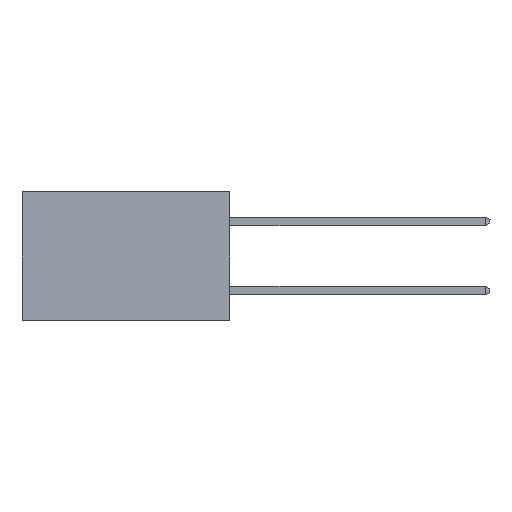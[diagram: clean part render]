
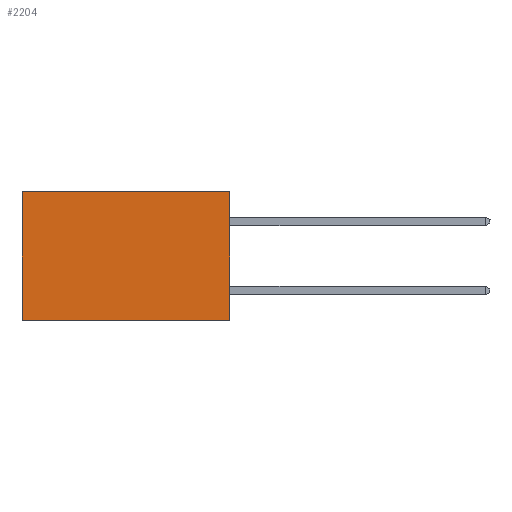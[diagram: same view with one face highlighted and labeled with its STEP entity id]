
A CAD part, left-side view. The second image highlights one B-rep face of the part: STEP entity #2204.
In plain terms, the highlighted planar face has unit normal (-1, 0, 0).
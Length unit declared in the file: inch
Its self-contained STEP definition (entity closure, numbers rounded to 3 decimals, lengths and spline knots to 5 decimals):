
#686 = CARTESIAN_POINT ( 'NONE',  ( 0.2615, 0., -0.37 ) ) ;
#1067 = CARTESIAN_POINT ( 'NONE',  ( 0.2615, 0.6, -0.37 ) ) ;
#1110 = VERTEX_POINT ( 'NONE', #8256 ) ;
#1580 = LINE ( 'NONE', #14676, #7391 ) ;
#1844 = ORIENTED_EDGE ( 'NONE', *, *, #2497, .F. ) ;
#1872 = EDGE_LOOP ( 'NONE', ( #11889, #1844, #11977, #18297 ) ) ;
#2204 = ADVANCED_FACE ( 'NONE', ( #3788 ), #12620, .F. ) ;
#2351 = LINE ( 'NONE', #4885, #16877 ) ;
#2497 = EDGE_CURVE ( 'NONE', #17773, #17491, #2351, .T. ) ;
#2535 = EDGE_CURVE ( 'NONE', #16802, #1110, #9160, .T. ) ;
#3332 = VECTOR ( 'NONE', #8151, 39.37008 ) ;
#3788 = FACE_OUTER_BOUND ( 'NONE', #1872, .T. ) ;
#4885 = CARTESIAN_POINT ( 'NONE',  ( 0.2615, 0., -0.37 ) ) ;
#5405 = EDGE_CURVE ( 'NONE', #1110, #17491, #5533, .T. ) ;
#5533 = LINE ( 'NONE', #14008, #3332 ) ;
#6440 = DIRECTION ( 'NONE',  ( 0., 1., 0. ) ) ;
#6583 = DIRECTION ( 'NONE',  ( 1., 0., 0. ) ) ;
#7236 = DIRECTION ( 'NONE',  ( 0., 0., -1. ) ) ;
#7391 = VECTOR ( 'NONE', #7236, 39.37008 ) ;
#7660 = VECTOR ( 'NONE', #17884, 39.37008 ) ;
#8151 = DIRECTION ( 'NONE',  ( 0., 0., -1. ) ) ;
#8256 = CARTESIAN_POINT ( 'NONE',  ( 0.2615, 0.6, 0. ) ) ;
#9160 = LINE ( 'NONE', #9415, #7660 ) ;
#9415 = CARTESIAN_POINT ( 'NONE',  ( 0.2615, 0., 0. ) ) ;
#10022 = AXIS2_PLACEMENT_3D ( 'NONE', #18288, #6583, #13656 ) ;
#11573 = EDGE_CURVE ( 'NONE', #16802, #17773, #1580, .T. ) ;
#11889 = ORIENTED_EDGE ( 'NONE', *, *, #5405, .T. ) ;
#11977 = ORIENTED_EDGE ( 'NONE', *, *, #11573, .F. ) ;
#12620 = PLANE ( 'NONE',  #10022 ) ;
#13656 = DIRECTION ( 'NONE',  ( 0., 0., -1. ) ) ;
#14008 = CARTESIAN_POINT ( 'NONE',  ( 0.2615, 0.6, -0.37 ) ) ;
#14676 = CARTESIAN_POINT ( 'NONE',  ( 0.2615, 0., -0.37 ) ) ;
#15879 = CARTESIAN_POINT ( 'NONE',  ( 0.2615, 0., 0. ) ) ;
#16802 = VERTEX_POINT ( 'NONE', #15879 ) ;
#16877 = VECTOR ( 'NONE', #6440, 39.37008 ) ;
#17491 = VERTEX_POINT ( 'NONE', #1067 ) ;
#17773 = VERTEX_POINT ( 'NONE', #686 ) ;
#17884 = DIRECTION ( 'NONE',  ( 0., 1., 0. ) ) ;
#18288 = CARTESIAN_POINT ( 'NONE',  ( 0.2615, 0., -0.37 ) ) ;
#18297 = ORIENTED_EDGE ( 'NONE', *, *, #2535, .T. ) ;
